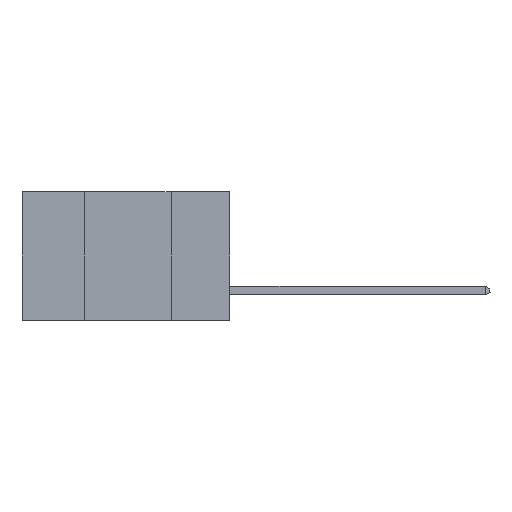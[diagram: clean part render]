
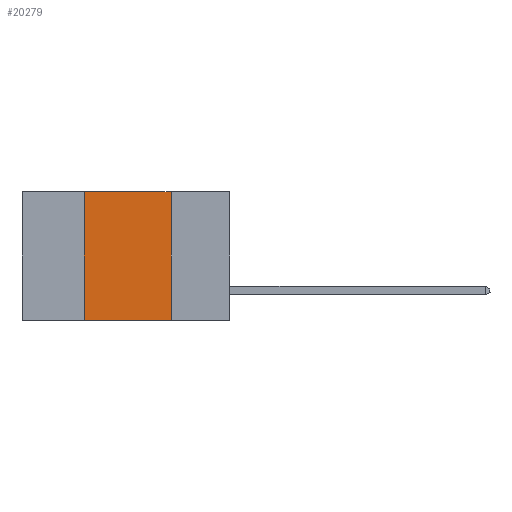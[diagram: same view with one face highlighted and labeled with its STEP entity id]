
A CAD part, left-side view. The second image highlights one B-rep face of the part: STEP entity #20279.
In plain terms, the highlighted planar face has unit normal (-1, 0, 0).
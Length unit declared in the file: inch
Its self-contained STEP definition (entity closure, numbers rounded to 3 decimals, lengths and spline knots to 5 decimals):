
#160 = VERTEX_POINT ( 'NONE', #1774 ) ;
#683 = DIRECTION ( 'NONE',  ( 0., 0., -1. ) ) ;
#730 = ORIENTED_EDGE ( 'NONE', *, *, #23250, .F. ) ;
#1746 = LINE ( 'NONE', #12467, #26031 ) ;
#1774 = CARTESIAN_POINT ( 'NONE',  ( 0., 0.42, 0. ) ) ;
#2122 = VERTEX_POINT ( 'NONE', #24976 ) ;
#3510 = FACE_OUTER_BOUND ( 'NONE', #14553, .T. ) ;
#4132 = AXIS2_PLACEMENT_3D ( 'NONE', #25302, #16905, #683 ) ;
#4769 = LINE ( 'NONE', #16719, #5773 ) ;
#5773 = VECTOR ( 'NONE', #20868, 39.37008 ) ;
#6834 = EDGE_CURVE ( 'NONE', #7357, #9282, #4769, .T. ) ;
#7357 = VERTEX_POINT ( 'NONE', #25649 ) ;
#7522 = ORIENTED_EDGE ( 'NONE', *, *, #6834, .T. ) ;
#7797 = VECTOR ( 'NONE', #13002, 39.37008 ) ;
#8440 = ORIENTED_EDGE ( 'NONE', *, *, #18930, .F. ) ;
#8487 = VECTOR ( 'NONE', #15500, 39.37008 ) ;
#9282 = VERTEX_POINT ( 'NONE', #19850 ) ;
#10734 = PLANE ( 'NONE',  #4132 ) ;
#12467 = CARTESIAN_POINT ( 'NONE',  ( 0., 0.6, 0. ) ) ;
#13002 = DIRECTION ( 'NONE',  ( 0., 0., 1. ) ) ;
#13004 = LINE ( 'NONE', #23239, #7797 ) ;
#14194 = DIRECTION ( 'NONE',  ( 0., -1., 0. ) ) ;
#14553 = EDGE_LOOP ( 'NONE', ( #20495, #730, #8440, #7522 ) ) ;
#15500 = DIRECTION ( 'NONE',  ( 0., 0., -1. ) ) ;
#16719 = CARTESIAN_POINT ( 'NONE',  ( 0., 0.6, -0.37 ) ) ;
#16905 = DIRECTION ( 'NONE',  ( 1., 0., 0. ) ) ;
#18551 = EDGE_CURVE ( 'NONE', #2122, #9282, #23016, .T. ) ;
#18930 = EDGE_CURVE ( 'NONE', #7357, #160, #13004, .T. ) ;
#19850 = CARTESIAN_POINT ( 'NONE',  ( 0., 0.17, -0.37 ) ) ;
#20279 = ADVANCED_FACE ( 'NONE', ( #3510 ), #10734, .F. ) ;
#20495 = ORIENTED_EDGE ( 'NONE', *, *, #18551, .F. ) ;
#20868 = DIRECTION ( 'NONE',  ( 0., -1., 0. ) ) ;
#23016 = LINE ( 'NONE', #25792, #8487 ) ;
#23239 = CARTESIAN_POINT ( 'NONE',  ( 0., 0.42, 0. ) ) ;
#23250 = EDGE_CURVE ( 'NONE', #160, #2122, #1746, .T. ) ;
#24976 = CARTESIAN_POINT ( 'NONE',  ( 0., 0.17, 0. ) ) ;
#25302 = CARTESIAN_POINT ( 'NONE',  ( 0., 0.6, 0. ) ) ;
#25649 = CARTESIAN_POINT ( 'NONE',  ( 0., 0.42, -0.37 ) ) ;
#25792 = CARTESIAN_POINT ( 'NONE',  ( 0., 0.17, 0. ) ) ;
#26031 = VECTOR ( 'NONE', #14194, 39.37008 ) ;
